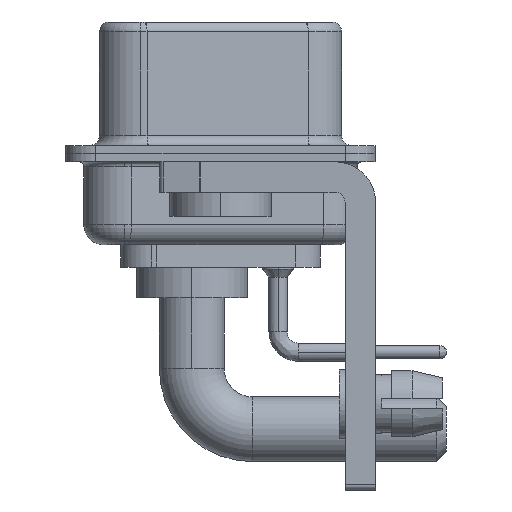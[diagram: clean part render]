
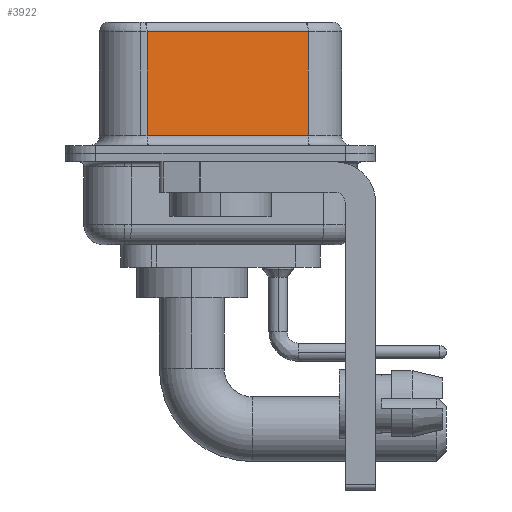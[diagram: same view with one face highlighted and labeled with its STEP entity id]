
A CAD part, left-side view. The second image highlights one B-rep face of the part: STEP entity #3922.
In plain terms, the highlighted planar face has unit normal (-0.985, -0.174, 0).
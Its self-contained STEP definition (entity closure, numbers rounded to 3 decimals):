
#797 = ORIENTED_EDGE ( 'NONE', *, *, #19586, .F. ) ;
#1520 = CARTESIAN_POINT ( 'NONE',  ( 5.132, -4.322, 6.52 ) ) ;
#1879 = CARTESIAN_POINT ( 'NONE',  ( 3.73, 3.628, 6.52 ) ) ;
#3038 = ORIENTED_EDGE ( 'NONE', *, *, #25168, .T. ) ;
#3401 = FACE_OUTER_BOUND ( 'NONE', #10078, .T. ) ;
#3922 = ADVANCED_FACE ( 'NONE', ( #3401 ), #7816, .F. ) ;
#4702 = VERTEX_POINT ( 'NONE', #9598 ) ;
#4742 = VECTOR ( 'NONE', #11930, 1000. ) ;
#4871 = VERTEX_POINT ( 'NONE', #16548 ) ;
#4964 = CARTESIAN_POINT ( 'NONE',  ( 3.73, 3.628, 0.9 ) ) ;
#5065 = ORIENTED_EDGE ( 'NONE', *, *, #20987, .T. ) ;
#5282 = VECTOR ( 'NONE', #24219, 1000. ) ;
#7488 = EDGE_CURVE ( 'NONE', #22679, #4702, #16311, .T. ) ;
#7816 = PLANE ( 'NONE',  #8920 ) ;
#7866 = DIRECTION ( 'NONE',  ( 0.174, -0.985, 0. ) ) ;
#8920 = AXIS2_PLACEMENT_3D ( 'NONE', #1520, #24147, #11967 ) ;
#9598 = CARTESIAN_POINT ( 'NONE',  ( 5.132, -4.322, 0.9 ) ) ;
#10016 = CARTESIAN_POINT ( 'NONE',  ( 5.132, -4.322, 0.9 ) ) ;
#10078 = EDGE_LOOP ( 'NONE', ( #797, #3038, #5065, #21483 ) ) ;
#10875 = LINE ( 'NONE', #25462, #18334 ) ;
#11930 = DIRECTION ( 'NONE',  ( 0., 0., -1. ) ) ;
#11967 = DIRECTION ( 'NONE',  ( -0.174, 0.985, 0. ) ) ;
#12722 = VERTEX_POINT ( 'NONE', #19074 ) ;
#14556 = VECTOR ( 'NONE', #7866, 1000. ) ;
#15298 = DIRECTION ( 'NONE',  ( 0., 0., -1. ) ) ;
#16311 = LINE ( 'NONE', #10016, #14556 ) ;
#16548 = CARTESIAN_POINT ( 'NONE',  ( 3.73, 3.628, 6.02 ) ) ;
#18334 = VECTOR ( 'NONE', #15298, 1000. ) ;
#19074 = CARTESIAN_POINT ( 'NONE',  ( 5.132, -4.322, 6.02 ) ) ;
#19586 = EDGE_CURVE ( 'NONE', #12722, #4702, #10875, .T. ) ;
#19818 = CARTESIAN_POINT ( 'NONE',  ( 5.132, -4.322, 6.02 ) ) ;
#20211 = LINE ( 'NONE', #19818, #5282 ) ;
#20987 = EDGE_CURVE ( 'NONE', #4871, #22679, #25725, .T. ) ;
#21483 = ORIENTED_EDGE ( 'NONE', *, *, #7488, .T. ) ;
#22679 = VERTEX_POINT ( 'NONE', #4964 ) ;
#24147 = DIRECTION ( 'NONE',  ( 0.985, 0.174, 0. ) ) ;
#24219 = DIRECTION ( 'NONE',  ( -0.174, 0.985, 0. ) ) ;
#25168 = EDGE_CURVE ( 'NONE', #12722, #4871, #20211, .T. ) ;
#25462 = CARTESIAN_POINT ( 'NONE',  ( 5.132, -4.322, 6.52 ) ) ;
#25725 = LINE ( 'NONE', #1879, #4742 ) ;
